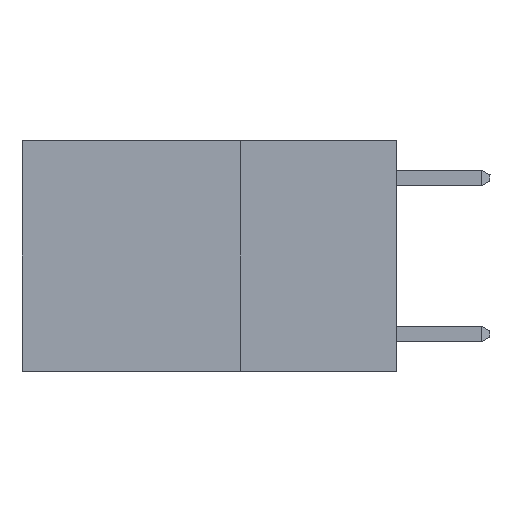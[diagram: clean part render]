
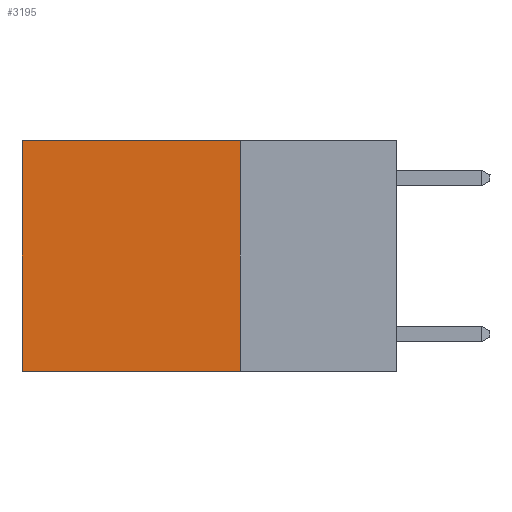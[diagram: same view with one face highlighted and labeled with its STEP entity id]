
A CAD part, left-side view. The second image highlights one B-rep face of the part: STEP entity #3195.
In plain terms, the highlighted planar face has unit normal (-1, 0, 0).
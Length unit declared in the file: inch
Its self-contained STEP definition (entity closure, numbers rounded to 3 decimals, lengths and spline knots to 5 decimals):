
#213 = CARTESIAN_POINT ( 'NONE',  ( 0.2625, 0.25, 0. ) ) ;
#261 = ORIENTED_EDGE ( 'NONE', *, *, #6026, .T. ) ;
#600 = ORIENTED_EDGE ( 'NONE', *, *, #5686, .F. ) ;
#686 = EDGE_CURVE ( 'NONE', #6378, #4005, #1549, .T. ) ;
#1014 = VECTOR ( 'NONE', #2520, 39.37008 ) ;
#1129 = CARTESIAN_POINT ( 'NONE',  ( 0.2625, 0.25, -0.37 ) ) ;
#1207 = LINE ( 'NONE', #3720, #3448 ) ;
#1479 = LINE ( 'NONE', #213, #5506 ) ;
#1549 = LINE ( 'NONE', #1129, #1014 ) ;
#1788 = ORIENTED_EDGE ( 'NONE', *, *, #686, .F. ) ;
#1827 = CARTESIAN_POINT ( 'NONE',  ( 0.2625, 0.6, 0. ) ) ;
#2450 = CARTESIAN_POINT ( 'NONE',  ( 0.2625, 0.6, -0.37 ) ) ;
#2520 = DIRECTION ( 'NONE',  ( 0., 1., 0. ) ) ;
#3092 = ORIENTED_EDGE ( 'NONE', *, *, #3418, .T. ) ;
#3195 = ADVANCED_FACE ( 'NONE', ( #4624 ), #4666, .F. ) ;
#3317 = VERTEX_POINT ( 'NONE', #5539 ) ;
#3418 = EDGE_CURVE ( 'NONE', #5200, #4005, #1207, .T. ) ;
#3448 = VECTOR ( 'NONE', #3769, 39.37008 ) ;
#3720 = CARTESIAN_POINT ( 'NONE',  ( 0.2625, 0.6, 0. ) ) ;
#3769 = DIRECTION ( 'NONE',  ( 0., 0., -1. ) ) ;
#3808 = CARTESIAN_POINT ( 'NONE',  ( 0.2625, 0.25, -0.37 ) ) ;
#3962 = AXIS2_PLACEMENT_3D ( 'NONE', #5892, #7093, #6487 ) ;
#4005 = VERTEX_POINT ( 'NONE', #2450 ) ;
#4092 = DIRECTION ( 'NONE',  ( 0., 0., -1. ) ) ;
#4624 = FACE_OUTER_BOUND ( 'NONE', #7805, .T. ) ;
#4666 = PLANE ( 'NONE',  #3962 ) ;
#4970 = VECTOR ( 'NONE', #5672, 39.37008 ) ;
#5200 = VERTEX_POINT ( 'NONE', #1827 ) ;
#5506 = VECTOR ( 'NONE', #4092, 39.37008 ) ;
#5539 = CARTESIAN_POINT ( 'NONE',  ( 0.2625, 0.25, 0. ) ) ;
#5672 = DIRECTION ( 'NONE',  ( 0., 1., 0. ) ) ;
#5686 = EDGE_CURVE ( 'NONE', #3317, #6378, #1479, .T. ) ;
#5745 = LINE ( 'NONE', #8327, #4970 ) ;
#5892 = CARTESIAN_POINT ( 'NONE',  ( 0.2625, 0.25, 0. ) ) ;
#6026 = EDGE_CURVE ( 'NONE', #3317, #5200, #5745, .T. ) ;
#6378 = VERTEX_POINT ( 'NONE', #3808 ) ;
#6487 = DIRECTION ( 'NONE',  ( 0., 0., -1. ) ) ;
#7093 = DIRECTION ( 'NONE',  ( 1., 0., 0. ) ) ;
#7805 = EDGE_LOOP ( 'NONE', ( #3092, #1788, #600, #261 ) ) ;
#8327 = CARTESIAN_POINT ( 'NONE',  ( 0.2625, 0.25, 0. ) ) ;
